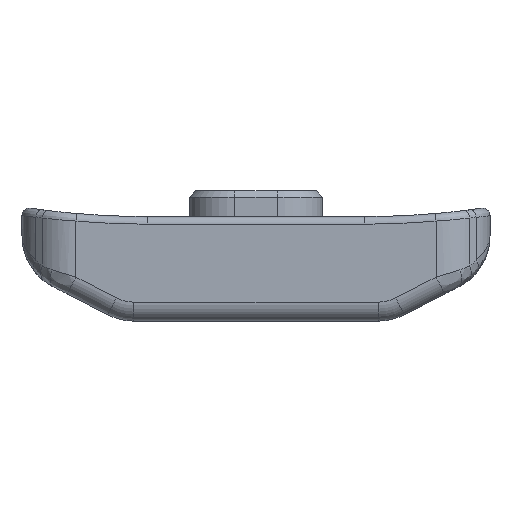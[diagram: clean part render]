
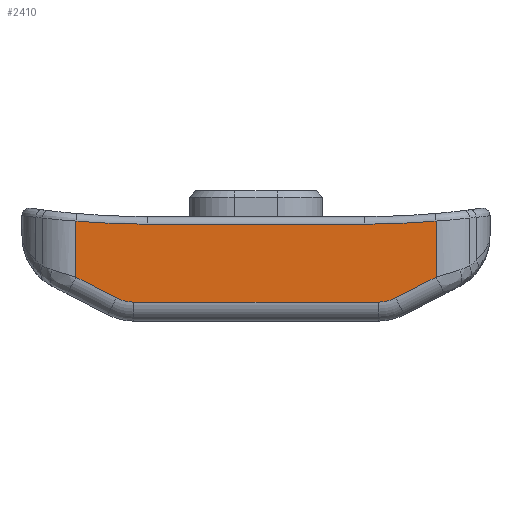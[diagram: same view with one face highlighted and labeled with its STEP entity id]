
A CAD part, front view. The second image highlights one B-rep face of the part: STEP entity #2410.
In plain terms, the highlighted planar face has unit normal (0, -1, 0).
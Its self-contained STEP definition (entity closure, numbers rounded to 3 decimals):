
#140=PLANE('',#2602);
#191=LINE('',#3739,#343);
#192=LINE('',#3743,#344);
#193=LINE('',#3745,#345);
#194=LINE('',#3749,#346);
#195=LINE('',#3753,#347);
#196=LINE('',#3755,#348);
#343=VECTOR('',#2947,10.);
#344=VECTOR('',#2952,10.);
#345=VECTOR('',#2953,10.);
#346=VECTOR('',#2956,10.);
#347=VECTOR('',#2959,10.);
#348=VECTOR('',#2960,10.);
#549=FACE_OUTER_BOUND('',#717,.T.);
#717=EDGE_LOOP('',(#1668,#1669,#1670,#1671,#1672,#1673,#1674,#1675,#1676,
#1677));
#896=CIRCLE('',#2593,2.);
#901=CIRCLE('',#2603,43.691);
#902=CIRCLE('',#2604,43.691);
#903=CIRCLE('',#2605,2.);
#1054=VERTEX_POINT('',#3712);
#1057=VERTEX_POINT('',#3717);
#1063=VERTEX_POINT('',#3738);
#1064=VERTEX_POINT('',#3742);
#1065=VERTEX_POINT('',#3744);
#1066=VERTEX_POINT('',#3746);
#1067=VERTEX_POINT('',#3748);
#1068=VERTEX_POINT('',#3750);
#1069=VERTEX_POINT('',#3752);
#1070=VERTEX_POINT('',#3754);
#1276=EDGE_CURVE('',#1057,#1054,#896,.T.);
#1286=EDGE_CURVE('',#1054,#1063,#191,.T.);
#1288=EDGE_CURVE('',#1064,#1057,#192,.T.);
#1289=EDGE_CURVE('',#1065,#1064,#193,.T.);
#1290=EDGE_CURVE('',#1066,#1065,#901,.T.);
#1291=EDGE_CURVE('',#1067,#1066,#194,.T.);
#1292=EDGE_CURVE('',#1068,#1067,#902,.T.);
#1293=EDGE_CURVE('',#1069,#1068,#195,.T.);
#1294=EDGE_CURVE('',#1070,#1069,#196,.T.);
#1295=EDGE_CURVE('',#1063,#1070,#903,.T.);
#1668=ORIENTED_EDGE('',*,*,#1276,.F.);
#1669=ORIENTED_EDGE('',*,*,#1288,.F.);
#1670=ORIENTED_EDGE('',*,*,#1289,.F.);
#1671=ORIENTED_EDGE('',*,*,#1290,.F.);
#1672=ORIENTED_EDGE('',*,*,#1291,.F.);
#1673=ORIENTED_EDGE('',*,*,#1292,.F.);
#1674=ORIENTED_EDGE('',*,*,#1293,.F.);
#1675=ORIENTED_EDGE('',*,*,#1294,.F.);
#1676=ORIENTED_EDGE('',*,*,#1295,.F.);
#1677=ORIENTED_EDGE('',*,*,#1286,.F.);
#2410=ADVANCED_FACE('',(#549),#140,.T.);
#2593=AXIS2_PLACEMENT_3D('',#3719,#2925,#2926);
#2602=AXIS2_PLACEMENT_3D('',#3741,#2950,#2951);
#2603=AXIS2_PLACEMENT_3D('',#3747,#2954,#2955);
#2604=AXIS2_PLACEMENT_3D('',#3751,#2957,#2958);
#2605=AXIS2_PLACEMENT_3D('',#3756,#2961,#2962);
#2925=DIRECTION('center_axis',(0.,1.,0.));
#2926=DIRECTION('ref_axis',(0.235,0.,-0.972));
#2947=DIRECTION('',(-1.,0.,0.));
#2950=DIRECTION('center_axis',(0.,-1.,0.));
#2951=DIRECTION('ref_axis',(0.,0.,-1.));
#2952=DIRECTION('',(-0.889,0.,-0.457));
#2953=DIRECTION('',(0.,0.,-1.));
#2954=DIRECTION('center_axis',(0.,-1.,0.));
#2955=DIRECTION('ref_axis',(0.043,0.,-0.999));
#2956=DIRECTION('',(1.,0.,0.));
#2957=DIRECTION('center_axis',(0.,-1.,0.));
#2958=DIRECTION('ref_axis',(-0.043,0.,-0.999));
#2959=DIRECTION('',(0.,0.,1.));
#2960=DIRECTION('',(-0.889,0.,0.457));
#2961=DIRECTION('center_axis',(0.,1.,0.));
#2962=DIRECTION('ref_axis',(-0.235,0.,-0.972));
#3712=CARTESIAN_POINT('',(-73.579,-35.5,-7.3));
#3717=CARTESIAN_POINT('',(-72.665,-35.5,-7.079));
#3719=CARTESIAN_POINT('Origin',(-73.579,-35.5,-5.3));
#3738=CARTESIAN_POINT('',(-86.421,-35.5,-7.3));
#3739=CARTESIAN_POINT('',(-86.25,-35.5,-7.3));
#3741=CARTESIAN_POINT('Origin',(-80.,-35.5,-4.89));
#3742=CARTESIAN_POINT('',(-70.536,-35.5,-5.985));
#3743=CARTESIAN_POINT('',(-75.444,-35.5,-8.507));
#3744=CARTESIAN_POINT('',(-70.536,-35.5,-3.039));
#3745=CARTESIAN_POINT('',(-70.536,-35.5,-4.368));
#3746=CARTESIAN_POINT('',(-74.287,-35.5,-3.2));
#3747=CARTESIAN_POINT('Origin',(-74.287,-35.5,40.491));
#3748=CARTESIAN_POINT('',(-85.713,-35.5,-3.2));
#3749=CARTESIAN_POINT('',(-80.,-35.5,-3.2));
#3750=CARTESIAN_POINT('',(-89.464,-35.5,-3.039));
#3751=CARTESIAN_POINT('Origin',(-85.713,-35.5,40.491));
#3752=CARTESIAN_POINT('',(-89.464,-35.5,-5.985));
#3753=CARTESIAN_POINT('',(-89.464,-35.5,-4.368));
#3754=CARTESIAN_POINT('',(-87.335,-35.5,-7.079));
#3755=CARTESIAN_POINT('',(-87.232,-35.5,-7.132));
#3756=CARTESIAN_POINT('Origin',(-86.421,-35.5,-5.3));
